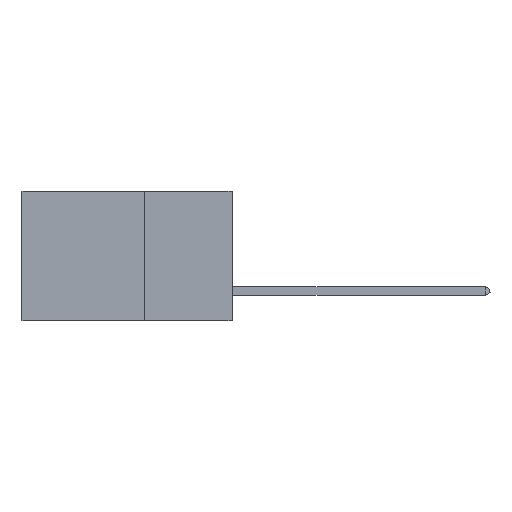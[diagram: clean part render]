
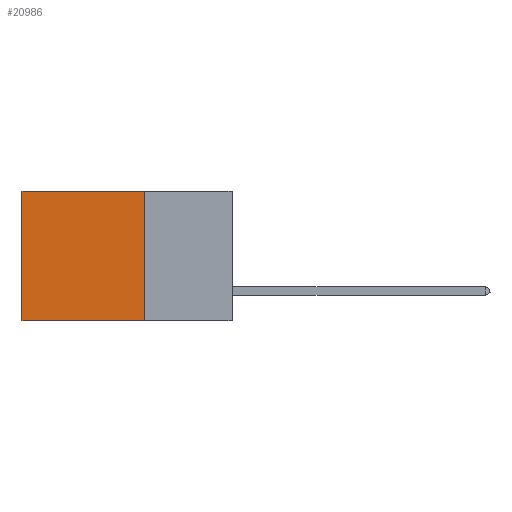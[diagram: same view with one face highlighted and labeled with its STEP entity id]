
A CAD part, left-side view. The second image highlights one B-rep face of the part: STEP entity #20986.
In plain terms, the highlighted planar face has unit normal (-1, 0, 0).
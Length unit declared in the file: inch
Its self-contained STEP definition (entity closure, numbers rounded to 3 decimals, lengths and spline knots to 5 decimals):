
#1224 = VECTOR ( 'NONE', #18532, 39.37008 ) ;
#2111 = CARTESIAN_POINT ( 'NONE',  ( 0.2875, 0.25, 0. ) ) ;
#3276 = VECTOR ( 'NONE', #16346, 39.37008 ) ;
#3645 = LINE ( 'NONE', #18474, #3276 ) ;
#4802 = CARTESIAN_POINT ( 'NONE',  ( 0.2875, 0.25, -0.37 ) ) ;
#5431 = VECTOR ( 'NONE', #17219, 39.37008 ) ;
#5783 = ORIENTED_EDGE ( 'NONE', *, *, #28437, .T. ) ;
#6129 = DIRECTION ( 'NONE',  ( 0., 0., -1. ) ) ;
#6528 = ORIENTED_EDGE ( 'NONE', *, *, #16185, .F. ) ;
#7504 = EDGE_CURVE ( 'NONE', #26609, #15919, #25489, .T. ) ;
#9558 = EDGE_LOOP ( 'NONE', ( #22841, #6528, #13079, #5783 ) ) ;
#9571 = VERTEX_POINT ( 'NONE', #13016 ) ;
#11029 = CARTESIAN_POINT ( 'NONE',  ( 0.2875, 0.6, 0. ) ) ;
#11948 = AXIS2_PLACEMENT_3D ( 'NONE', #17270, #28312, #6129 ) ;
#13016 = CARTESIAN_POINT ( 'NONE',  ( 0.2875, 0.6, -0.37 ) ) ;
#13079 = ORIENTED_EDGE ( 'NONE', *, *, #7504, .F. ) ;
#15517 = VERTEX_POINT ( 'NONE', #11029 ) ;
#15530 = VECTOR ( 'NONE', #26149, 39.37008 ) ;
#15919 = VERTEX_POINT ( 'NONE', #27387 ) ;
#16185 = EDGE_CURVE ( 'NONE', #15919, #9571, #25350, .T. ) ;
#16346 = DIRECTION ( 'NONE',  ( 0., 0., -1. ) ) ;
#17082 = PLANE ( 'NONE',  #11948 ) ;
#17219 = DIRECTION ( 'NONE',  ( 0., 1., 0. ) ) ;
#17270 = CARTESIAN_POINT ( 'NONE',  ( 0.2875, 0.25, 0. ) ) ;
#18474 = CARTESIAN_POINT ( 'NONE',  ( 0.2875, 0.6, 0. ) ) ;
#18532 = DIRECTION ( 'NONE',  ( 0., 1., 0. ) ) ;
#19947 = FACE_OUTER_BOUND ( 'NONE', #9558, .T. ) ;
#20925 = EDGE_CURVE ( 'NONE', #15517, #9571, #3645, .T. ) ;
#20986 = ADVANCED_FACE ( 'NONE', ( #19947 ), #17082, .F. ) ;
#22841 = ORIENTED_EDGE ( 'NONE', *, *, #20925, .T. ) ;
#23116 = LINE ( 'NONE', #24077, #5431 ) ;
#24077 = CARTESIAN_POINT ( 'NONE',  ( 0.2875, 0.25, 0. ) ) ;
#25350 = LINE ( 'NONE', #4802, #1224 ) ;
#25489 = LINE ( 'NONE', #2111, #15530 ) ;
#26149 = DIRECTION ( 'NONE',  ( 0., 0., -1. ) ) ;
#26609 = VERTEX_POINT ( 'NONE', #26662 ) ;
#26662 = CARTESIAN_POINT ( 'NONE',  ( 0.2875, 0.25, 0. ) ) ;
#27387 = CARTESIAN_POINT ( 'NONE',  ( 0.2875, 0.25, -0.37 ) ) ;
#28312 = DIRECTION ( 'NONE',  ( 1., 0., 0. ) ) ;
#28437 = EDGE_CURVE ( 'NONE', #26609, #15517, #23116, .T. ) ;
